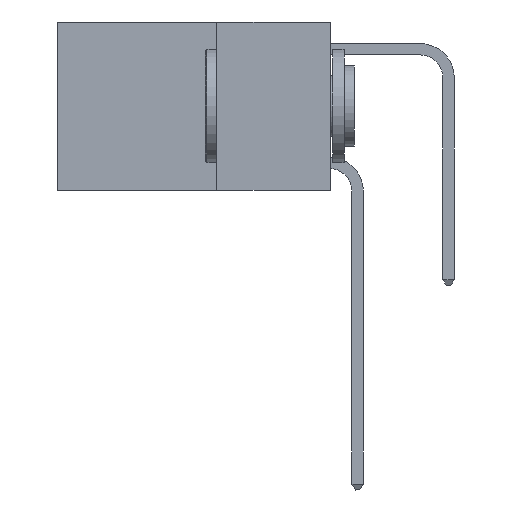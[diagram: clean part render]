
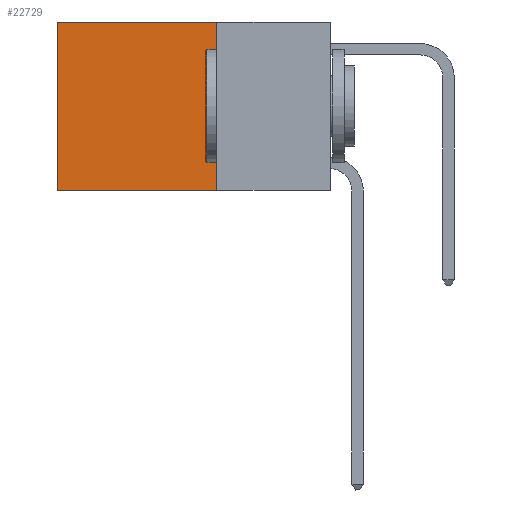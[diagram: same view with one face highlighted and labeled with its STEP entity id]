
A CAD part, left-side view. The second image highlights one B-rep face of the part: STEP entity #22729.
In plain terms, the highlighted planar face has unit normal (-1, 0, 0).
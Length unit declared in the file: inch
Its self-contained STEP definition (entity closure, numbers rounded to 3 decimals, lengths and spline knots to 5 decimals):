
#11 = CARTESIAN_POINT ( 'NONE',  ( 0.2625, 0.6, -0.37 ) ) ;
#1991 = VECTOR ( 'NONE', #29824, 39.37008 ) ;
#3595 = LINE ( 'NONE', #6687, #30492 ) ;
#6331 = VECTOR ( 'NONE', #14015, 39.37008 ) ;
#6687 = CARTESIAN_POINT ( 'NONE',  ( 0.2625, 0.25, 0. ) ) ;
#10442 = ORIENTED_EDGE ( 'NONE', *, *, #11266, .F. ) ;
#10579 = EDGE_CURVE ( 'NONE', #15593, #16750, #19183, .T. ) ;
#11266 = EDGE_CURVE ( 'NONE', #30595, #15593, #3595, .T. ) ;
#11430 = CARTESIAN_POINT ( 'NONE',  ( 0.2625, 0.6, 0. ) ) ;
#11692 = LINE ( 'NONE', #22196, #17734 ) ;
#12199 = DIRECTION ( 'NONE',  ( 0., 1., 0. ) ) ;
#14015 = DIRECTION ( 'NONE',  ( 0., 1., 0. ) ) ;
#14081 = DIRECTION ( 'NONE',  ( 0., 0., -1. ) ) ;
#14789 = ORIENTED_EDGE ( 'NONE', *, *, #29448, .T. ) ;
#15593 = VERTEX_POINT ( 'NONE', #19606 ) ;
#16750 = VERTEX_POINT ( 'NONE', #11 ) ;
#17461 = PLANE ( 'NONE',  #19924 ) ;
#17734 = VECTOR ( 'NONE', #12199, 39.37008 ) ;
#18091 = EDGE_LOOP ( 'NONE', ( #33184, #18876, #10442, #14789 ) ) ;
#18876 = ORIENTED_EDGE ( 'NONE', *, *, #10579, .F. ) ;
#19183 = LINE ( 'NONE', #29654, #6331 ) ;
#19606 = CARTESIAN_POINT ( 'NONE',  ( 0.2625, 0.25, -0.37 ) ) ;
#19924 = AXIS2_PLACEMENT_3D ( 'NONE', #20218, #33596, #32910 ) ;
#20218 = CARTESIAN_POINT ( 'NONE',  ( 0.2625, 0.25, 0. ) ) ;
#20711 = VERTEX_POINT ( 'NONE', #21773 ) ;
#21557 = CARTESIAN_POINT ( 'NONE',  ( 0.2625, 0.25, 0. ) ) ;
#21773 = CARTESIAN_POINT ( 'NONE',  ( 0.2625, 0.6, 0. ) ) ;
#22196 = CARTESIAN_POINT ( 'NONE',  ( 0.2625, 0.25, 0. ) ) ;
#22729 = ADVANCED_FACE ( 'NONE', ( #23147 ), #17461, .F. ) ;
#23147 = FACE_OUTER_BOUND ( 'NONE', #18091, .T. ) ;
#24495 = LINE ( 'NONE', #11430, #1991 ) ;
#29448 = EDGE_CURVE ( 'NONE', #30595, #20711, #11692, .T. ) ;
#29654 = CARTESIAN_POINT ( 'NONE',  ( 0.2625, 0.25, -0.37 ) ) ;
#29824 = DIRECTION ( 'NONE',  ( 0., 0., -1. ) ) ;
#30423 = EDGE_CURVE ( 'NONE', #20711, #16750, #24495, .T. ) ;
#30492 = VECTOR ( 'NONE', #14081, 39.37008 ) ;
#30595 = VERTEX_POINT ( 'NONE', #21557 ) ;
#32910 = DIRECTION ( 'NONE',  ( 0., 0., -1. ) ) ;
#33184 = ORIENTED_EDGE ( 'NONE', *, *, #30423, .T. ) ;
#33596 = DIRECTION ( 'NONE',  ( 1., 0., 0. ) ) ;
